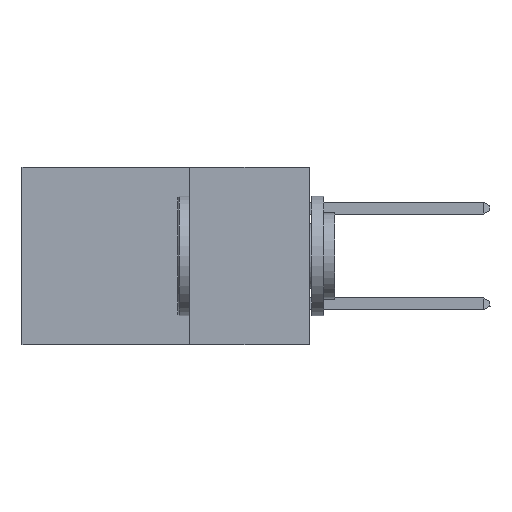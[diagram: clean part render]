
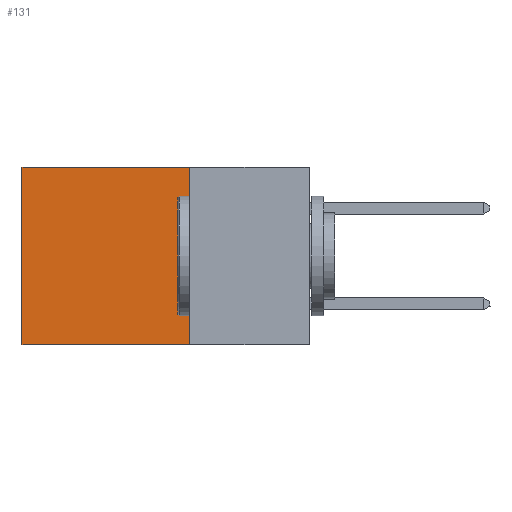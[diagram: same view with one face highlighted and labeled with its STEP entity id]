
A CAD part, left-side view. The second image highlights one B-rep face of the part: STEP entity #131.
In plain terms, the highlighted planar face has unit normal (-1, 0, 0).
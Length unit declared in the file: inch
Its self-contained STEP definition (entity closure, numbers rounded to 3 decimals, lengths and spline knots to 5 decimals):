
#131 = ADVANCED_FACE ( 'NONE', ( #7192 ), #4589, .F. ) ;
#261 = LINE ( 'NONE', #1951, #7950 ) ;
#420 = VERTEX_POINT ( 'NONE', #1982 ) ;
#438 = DIRECTION ( 'NONE',  ( 0., 0., -1. ) ) ;
#623 = EDGE_CURVE ( 'NONE', #3103, #1342, #6576, .T. ) ;
#1332 = VERTEX_POINT ( 'NONE', #8454 ) ;
#1342 = VERTEX_POINT ( 'NONE', #7840 ) ;
#1344 = CARTESIAN_POINT ( 'NONE',  ( 0.2875, 0.25, 0. ) ) ;
#1404 = DIRECTION ( 'NONE',  ( 0., 1., 0. ) ) ;
#1951 = CARTESIAN_POINT ( 'NONE',  ( 0.2875, 0.6, 0. ) ) ;
#1982 = CARTESIAN_POINT ( 'NONE',  ( 0.2875, 0.25, -0.37 ) ) ;
#2100 = EDGE_LOOP ( 'NONE', ( #6932, #3535, #7333, #7545 ) ) ;
#2597 = EDGE_CURVE ( 'NONE', #3103, #420, #8616, .T. ) ;
#3103 = VERTEX_POINT ( 'NONE', #6045 ) ;
#3535 = ORIENTED_EDGE ( 'NONE', *, *, #6343, .F. ) ;
#4589 = PLANE ( 'NONE',  #4784 ) ;
#4720 = VECTOR ( 'NONE', #6339, 39.37008 ) ;
#4784 = AXIS2_PLACEMENT_3D ( 'NONE', #5647, #7308, #7329 ) ;
#5050 = VECTOR ( 'NONE', #438, 39.37008 ) ;
#5297 = CARTESIAN_POINT ( 'NONE',  ( 0.2875, 0.25, -0.37 ) ) ;
#5582 = EDGE_CURVE ( 'NONE', #1342, #1332, #261, .T. ) ;
#5647 = CARTESIAN_POINT ( 'NONE',  ( 0.2875, 0.25, 0. ) ) ;
#5858 = LINE ( 'NONE', #5297, #8778 ) ;
#6045 = CARTESIAN_POINT ( 'NONE',  ( 0.2875, 0.25, 0. ) ) ;
#6339 = DIRECTION ( 'NONE',  ( 0., 1., 0. ) ) ;
#6343 = EDGE_CURVE ( 'NONE', #420, #1332, #5858, .T. ) ;
#6576 = LINE ( 'NONE', #7122, #4720 ) ;
#6932 = ORIENTED_EDGE ( 'NONE', *, *, #5582, .T. ) ;
#7122 = CARTESIAN_POINT ( 'NONE',  ( 0.2875, 0.25, 0. ) ) ;
#7192 = FACE_OUTER_BOUND ( 'NONE', #2100, .T. ) ;
#7308 = DIRECTION ( 'NONE',  ( 1., 0., 0. ) ) ;
#7329 = DIRECTION ( 'NONE',  ( 0., 0., -1. ) ) ;
#7333 = ORIENTED_EDGE ( 'NONE', *, *, #2597, .F. ) ;
#7545 = ORIENTED_EDGE ( 'NONE', *, *, #623, .T. ) ;
#7840 = CARTESIAN_POINT ( 'NONE',  ( 0.2875, 0.6, 0. ) ) ;
#7950 = VECTOR ( 'NONE', #9172, 39.37008 ) ;
#8454 = CARTESIAN_POINT ( 'NONE',  ( 0.2875, 0.6, -0.37 ) ) ;
#8616 = LINE ( 'NONE', #1344, #5050 ) ;
#8778 = VECTOR ( 'NONE', #1404, 39.37008 ) ;
#9172 = DIRECTION ( 'NONE',  ( 0., 0., -1. ) ) ;
